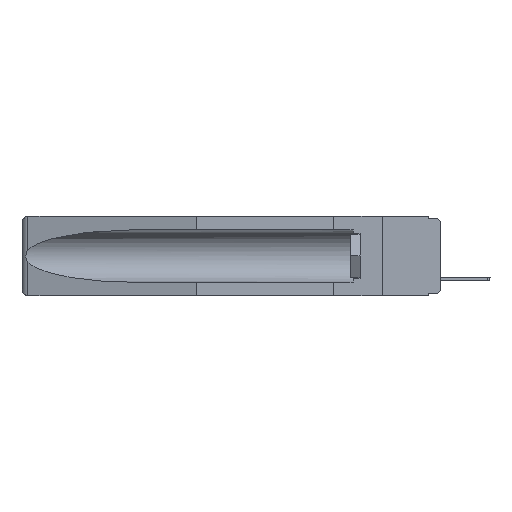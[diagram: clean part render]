
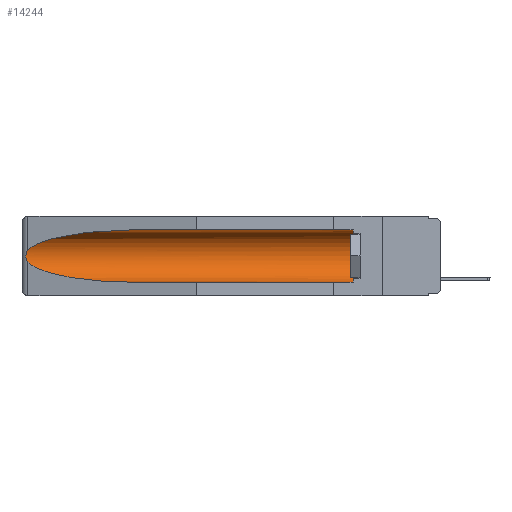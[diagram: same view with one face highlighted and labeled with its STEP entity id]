
A CAD part, left-side view. The second image highlights one B-rep face of the part: STEP entity #14244.
In plain terms, the highlighted cylindrical face has radius 2.857 mm (diameter 5.715 mm), a partial arc.
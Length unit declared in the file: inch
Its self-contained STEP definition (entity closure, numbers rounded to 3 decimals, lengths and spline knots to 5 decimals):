
#141 =( BOUNDED_CURVE ( )  B_SPLINE_CURVE ( 3, ( #2614, #11514, #1052, #901 ),
 .UNSPECIFIED., .F., .F. ) 
 B_SPLINE_CURVE_WITH_KNOTS ( ( 4, 4 ),
 ( 0.1948, 1.5708 ),
 .UNSPECIFIED. ) 
 CURVE ( )  GEOMETRIC_REPRESENTATION_ITEM ( )  RATIONAL_B_SPLINE_CURVE ( ( 1., 0.848, 0.848, 1. ) ) 
 REPRESENTATION_ITEM ( '' )  );
#504 = ORIENTED_EDGE ( 'NONE', *, *, #13742, .T. ) ;
#901 = CARTESIAN_POINT ( 'NONE',  ( 0.155, 1.07973, -0.284 ) ) ;
#1052 = CARTESIAN_POINT ( 'NONE',  ( 0.21114, 1.30732, -0.284 ) ) ;
#1410 = DIRECTION ( 'NONE',  ( 0., 1., 0. ) ) ;
#1422 = VERTEX_POINT ( 'NONE', #2436 ) ;
#2267 = CARTESIAN_POINT ( 'NONE',  ( 0.2673, 1.53269, -0.17917 ) ) ;
#2327 = VECTOR ( 'NONE', #3571, 39.37008 ) ;
#2346 = CARTESIAN_POINT ( 'NONE',  ( 0.26537, 1.52718, -0.14972 ) ) ;
#2436 = CARTESIAN_POINT ( 'NONE',  ( 0.26537, 1.52718, -0.19328 ) ) ;
#2614 = CARTESIAN_POINT ( 'NONE',  ( 0.26537, 1.52718, -0.19328 ) ) ;
#2734 = EDGE_CURVE ( 'NONE', #3035, #1422, #20447, .T. ) ;
#3035 = VERTEX_POINT ( 'NONE', #13729 ) ;
#3324 = CARTESIAN_POINT ( 'NONE',  ( 0.155, -0.30754, -0.059 ) ) ;
#3397 = EDGE_LOOP ( 'NONE', ( #13102, #5037, #15991, #17056, #504, #16113 ) ) ;
#3571 = DIRECTION ( 'NONE',  ( 0., 1., 0. ) ) ;
#3845 = VERTEX_POINT ( 'NONE', #16354 ) ;
#4666 = VERTEX_POINT ( 'NONE', #16471 ) ;
#5037 = ORIENTED_EDGE ( 'NONE', *, *, #2734, .T. ) ;
#5911 = FACE_OUTER_BOUND ( 'NONE', #3397, .T. ) ;
#5928 = CARTESIAN_POINT ( 'NONE',  ( 0.2673, 1.5327, -0.16383 ) ) ;
#5996 = CARTESIAN_POINT ( 'NONE',  ( 0.2675, 1.53308, -0.16763 ) ) ;
#6551 = EDGE_CURVE ( 'NONE', #1422, #16571, #141, .T. ) ;
#6786 = CARTESIAN_POINT ( 'NONE',  ( 0.25451, 1.48313, -0.09465 ) ) ;
#7039 = CIRCLE ( 'NONE', #16138, 0.1125 ) ;
#7237 = DIRECTION ( 'NONE',  ( 0., 1., 0. ) ) ;
#7616 = CARTESIAN_POINT ( 'NONE',  ( 0.26597, 1.5296, -0.19026 ) ) ;
#8107 = CYLINDRICAL_SURFACE ( 'NONE', #13262, 0.1125 ) ;
#9061 = CARTESIAN_POINT ( 'NONE',  ( 0.155, 0.126, -0.059 ) ) ;
#9446 = CARTESIAN_POINT ( 'NONE',  ( 0.26537, 1.52718, -0.19328 ) ) ;
#9953 = CARTESIAN_POINT ( 'NONE',  ( 0.155, 0.126, -0.1715 ) ) ;
#10181 = CARTESIAN_POINT ( 'NONE',  ( 0.155, 1.07973, -0.059 ) ) ;
#11392 = LINE ( 'NONE', #22534, #16945 ) ;
#11514 = CARTESIAN_POINT ( 'NONE',  ( 0.25451, 1.48313, -0.24835 ) ) ;
#11806 = EDGE_CURVE ( 'NONE', #16794, #3845, #20635, .T. ) ;
#12290 = EDGE_CURVE ( 'NONE', #3845, #3035, #21195, .T. ) ;
#12954 = CARTESIAN_POINT ( 'NONE',  ( 0.26655, 1.53094, -0.18657 ) ) ;
#13102 = ORIENTED_EDGE ( 'NONE', *, *, #12290, .T. ) ;
#13262 = AXIS2_PLACEMENT_3D ( 'NONE', #19160, #7237, #15731 ) ;
#13468 = DIRECTION ( 'NONE',  ( 0., -1., 0. ) ) ;
#13621 = DIRECTION ( 'NONE',  ( 0., 0., 1. ) ) ;
#13729 = CARTESIAN_POINT ( 'NONE',  ( 0.26537, 1.52718, -0.14972 ) ) ;
#13742 = EDGE_CURVE ( 'NONE', #4666, #16794, #7039, .T. ) ;
#13914 = CARTESIAN_POINT ( 'NONE',  ( 0.26537, 1.52718, -0.14972 ) ) ;
#14244 = ADVANCED_FACE ( 'NONE', ( #5911 ), #8107, .F. ) ;
#14597 = CARTESIAN_POINT ( 'NONE',  ( 0.2675, 1.53308, -0.17534 ) ) ;
#14748 = CARTESIAN_POINT ( 'NONE',  ( 0.26654, 1.53092, -0.15636 ) ) ;
#15717 = CARTESIAN_POINT ( 'NONE',  ( 0.21114, 1.30732, -0.059 ) ) ;
#15731 = DIRECTION ( 'NONE',  ( 0., 0., 1. ) ) ;
#15991 = ORIENTED_EDGE ( 'NONE', *, *, #6551, .T. ) ;
#16113 = ORIENTED_EDGE ( 'NONE', *, *, #11806, .T. ) ;
#16138 = AXIS2_PLACEMENT_3D ( 'NONE', #9953, #13468, #13621 ) ;
#16354 = CARTESIAN_POINT ( 'NONE',  ( 0.155, 1.07973, -0.059 ) ) ;
#16471 = CARTESIAN_POINT ( 'NONE',  ( 0.155, 0.126, -0.284 ) ) ;
#16571 = VERTEX_POINT ( 'NONE', #17758 ) ;
#16794 = VERTEX_POINT ( 'NONE', #9061 ) ;
#16945 = VECTOR ( 'NONE', #1410, 39.37008 ) ;
#17056 = ORIENTED_EDGE ( 'NONE', *, *, #22457, .F. ) ;
#17758 = CARTESIAN_POINT ( 'NONE',  ( 0.155, 1.07973, -0.284 ) ) ;
#18211 = CARTESIAN_POINT ( 'NONE',  ( 0.26597, 1.52961, -0.15275 ) ) ;
#19160 = CARTESIAN_POINT ( 'NONE',  ( 0.155, -0.30754, -0.1715 ) ) ;
#20447 = B_SPLINE_CURVE_WITH_KNOTS ( 'NONE', 3,
 ( #2346, #18211, #14748, #5928, #5996, #14597, #2267, #12954, #7616, #9446 ),
 .UNSPECIFIED., .F., .F.,
 ( 4, 2, 2, 2, 4 ),
 ( 0., 0.00029, 0.00058, 0.00087, 0.00117 ),
 .UNSPECIFIED. ) ;
#20635 = LINE ( 'NONE', #3324, #2327 ) ;
#21195 =( BOUNDED_CURVE ( )  B_SPLINE_CURVE ( 3, ( #10181, #15717, #6786, #13914 ),
 .UNSPECIFIED., .F., .T. ) 
 B_SPLINE_CURVE_WITH_KNOTS ( ( 4, 4 ),
 ( 4.71239, 6.08839 ),
 .UNSPECIFIED. ) 
 CURVE ( )  GEOMETRIC_REPRESENTATION_ITEM ( )  RATIONAL_B_SPLINE_CURVE ( ( 1., 0.848, 0.848, 1. ) ) 
 REPRESENTATION_ITEM ( '' )  );
#22457 = EDGE_CURVE ( 'NONE', #4666, #16571, #11392, .T. ) ;
#22534 = CARTESIAN_POINT ( 'NONE',  ( 0.155, -0.30754, -0.284 ) ) ;
